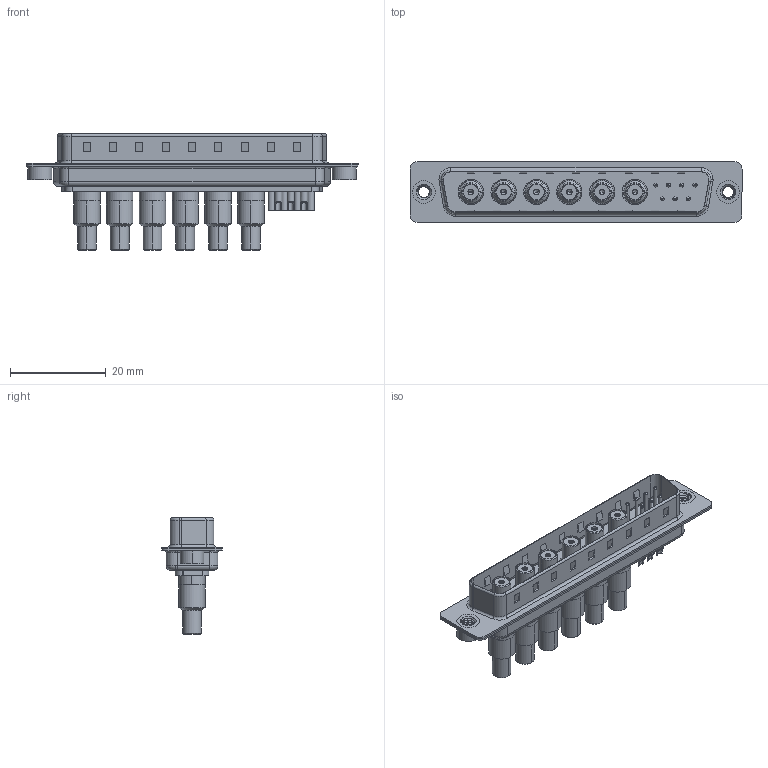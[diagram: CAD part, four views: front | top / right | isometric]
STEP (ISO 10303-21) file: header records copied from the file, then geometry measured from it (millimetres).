
FILE_DESCRIPTION (( 'STEP AP203' ), '1' );
FILE_NAME ('627-13W6622-7TA.STEP', '2019-05-28T21:42:29', ( '' ), ( '' ), 'SwSTEP 2.0', 'SolidWorks 2016', '' );
FILE_SCHEMA (( 'CONFIG_CONTROL_DESIGN' ));
Length unit declared in the file: millimetre
Products named in the file (15): 627Combo Threaded Rivet_2; 627Combo Threaded Rivet_A; 627Combo Shell Front_37 Contacts; 627Combo Contact Row 1_22; Co-Ax Jack_Solder Cup Tail; 627Combo Contact Row 2_22; Insulator Socket; 627-13W6622-7TA; Insulator Socket 2; Locking Collar; Socket_Solder Cup; Solder Cover; 627Combo Housing_13W6; Co-Ax Jack Assy_SC; 627Combo Shell Rear_37 Contacts
Assembly tree (24 placements, depth 3):
  627-13W6622-7TA
    627Combo Housing_13W6
    627Combo Shell Rear_37 Contacts
    627Combo Shell Front_37 Contacts
    627Combo Threaded Rivet_A
    Co-Ax Jack Assy_SC  x6
      Co-Ax Jack_Solder Cup Tail
      Insulator Socket
      Insulator Socket 2
      Locking Collar
      Socket_Solder Cup
      Solder Cover
    627Combo Threaded Rivet_2
    627Combo Contact Row 1_22  x4
    627Combo Contact Row 2_22  x3
Bounding box: 69.3 x 12.6 x 24.3 mm (x, y, z)
Volume: 4542.5 mm3; surface area: 14133.8 mm2
Topology: 48 solids, 48 shells, 1450 faces, 3376 edges, 2077 vertices
Faces by surface type: cylinder 638, plane 506, torus 144, cone 144, bspline 18
Entity records: 25243 total; most frequent: CARTESIAN_POINT 6944, DIRECTION 3603, ORIENTED_EDGE 3302, EDGE_CURVE 1651, AXIS2_PLACEMENT_3D 1365, VERTEX_POINT 1042, LINE 873, VECTOR 873
